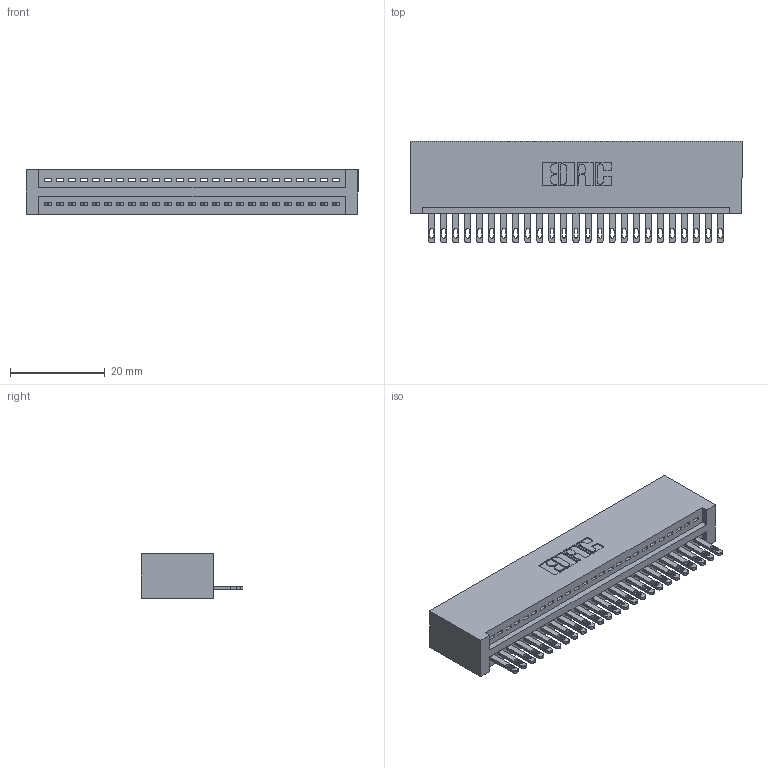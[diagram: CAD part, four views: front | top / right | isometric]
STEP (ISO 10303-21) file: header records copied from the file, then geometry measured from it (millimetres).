
FILE_DESCRIPTION (( 'STEP AP203' ), '1' );
FILE_NAME ('345-025-500-101.STEP', '2018-08-21T10:10:05', ( '' ), ( '' ), 'SwSTEP 2.0', 'SolidWorks 2016', '' );
FILE_SCHEMA (( 'CONFIG_CONTROL_DESIGN' ));
Length unit declared in the file: inch
Products named in the file (3): 345-025-500-101; 345 Part_No Mounting Lugs; 345-292-001_345-293-100
Assembly tree (26 placements, depth 2):
  345-025-500-101
    345 Part_No Mounting Lugs
    345-292-001_345-293-100  x25
Bounding box: 70.1 x 21.51 x 9.4 mm (x, y, z)
Volume: 7119.1 mm3; surface area: 9475.9 mm2
Topology: 26 solids, 26 shells, 1468 faces, 4517 edges, 3010 vertices
Faces by surface type: plane 926, cylinder 542
Entity records: 20757 total; most frequent: CARTESIAN_POINT 3603, ORIENTED_EDGE 3562, DIRECTION 3167, EDGE_CURVE 1781, VECTOR 1553, LINE 1553, VERTEX_POINT 1186, AXIS2_PLACEMENT_3D 807
